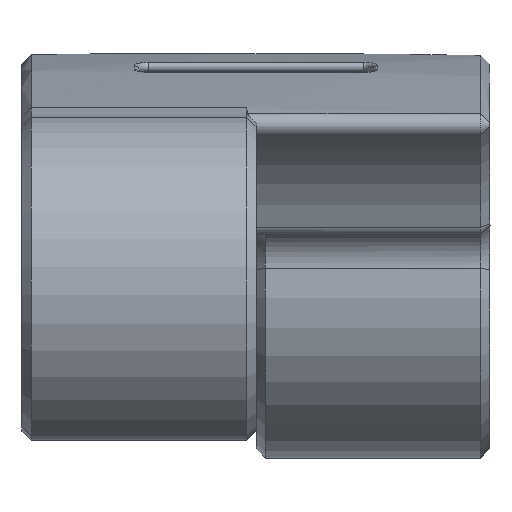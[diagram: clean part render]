
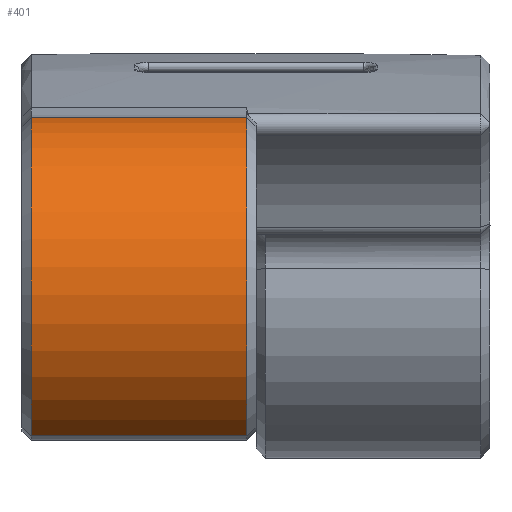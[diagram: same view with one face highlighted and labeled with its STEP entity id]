
A CAD part, front view. The second image highlights one B-rep face of the part: STEP entity #401.
In plain terms, the highlighted cylindrical face has radius 14.583 mm (diameter 29.165 mm), a partial arc.
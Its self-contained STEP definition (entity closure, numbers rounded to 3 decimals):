
#82 = DIRECTION ( 'NONE',  ( -1., 0., 0. ) ) ;
#241 = CYLINDRICAL_SURFACE ( 'NONE', #3236, 14.583 ) ;
#313 = CARTESIAN_POINT ( 'NONE',  ( -459.696, -70.336, 0.8 ) ) ;
#401 = ADVANCED_FACE ( 'NONE', ( #669 ), #241, .T. ) ;
#600 = DIRECTION ( 'NONE',  ( 0., 0., 1. ) ) ;
#618 = DIRECTION ( 'NONE',  ( 1., 0., 0. ) ) ;
#637 = VECTOR ( 'NONE', #3284, 1000. ) ;
#669 = FACE_OUTER_BOUND ( 'NONE', #1401, .T. ) ;
#715 = DIRECTION ( 'NONE',  ( 1., 0., 0. ) ) ;
#960 = ORIENTED_EDGE ( 'NONE', *, *, #1459, .F. ) ;
#1144 = DIRECTION ( 'NONE',  ( 0., 0., 1. ) ) ;
#1326 = CARTESIAN_POINT ( 'NONE',  ( -459.696, -77.575, -11.858 ) ) ;
#1401 = EDGE_LOOP ( 'NONE', ( #960, #3217, #1725, #2146 ) ) ;
#1449 = CARTESIAN_POINT ( 'NONE',  ( -445.481, -70.336, 0.8 ) ) ;
#1459 = EDGE_CURVE ( 'NONE', #3548, #3424, #3009, .T. ) ;
#1602 = VECTOR ( 'NONE', #715, 1000. ) ;
#1684 = EDGE_CURVE ( 'NONE', #3424, #3173, #1743, .T. ) ;
#1720 = DIRECTION ( 'NONE',  ( 1., 0., 0. ) ) ;
#1721 = CARTESIAN_POINT ( 'NONE',  ( -463.881, -70.336, 0.8 ) ) ;
#1725 = ORIENTED_EDGE ( 'NONE', *, *, #2529, .F. ) ;
#1743 = LINE ( 'NONE', #1326, #637 ) ;
#1800 = AXIS2_PLACEMENT_3D ( 'NONE', #1721, #82, #600 ) ;
#2042 = CIRCLE ( 'NONE', #1800, 14.583 ) ;
#2054 = AXIS2_PLACEMENT_3D ( 'NONE', #1449, #618, #2581 ) ;
#2146 = ORIENTED_EDGE ( 'NONE', *, *, #1684, .F. ) ;
#2283 = VERTEX_POINT ( 'NONE', #3160 ) ;
#2372 = CARTESIAN_POINT ( 'NONE',  ( -445.481, -69.39, 15.352 ) ) ;
#2411 = CARTESIAN_POINT ( 'NONE',  ( -454.681, -69.39, 15.352 ) ) ;
#2529 = EDGE_CURVE ( 'NONE', #3173, #2283, #2042, .T. ) ;
#2532 = LINE ( 'NONE', #2411, #1602 ) ;
#2581 = DIRECTION ( 'NONE',  ( 0., 0., 1. ) ) ;
#2991 = CARTESIAN_POINT ( 'NONE',  ( -445.481, -77.575, -11.858 ) ) ;
#3000 = CARTESIAN_POINT ( 'NONE',  ( -463.881, -77.575, -11.858 ) ) ;
#3009 = CIRCLE ( 'NONE', #2054, 14.583 ) ;
#3160 = CARTESIAN_POINT ( 'NONE',  ( -463.881, -69.39, 15.352 ) ) ;
#3173 = VERTEX_POINT ( 'NONE', #3000 ) ;
#3217 = ORIENTED_EDGE ( 'NONE', *, *, #3421, .F. ) ;
#3236 = AXIS2_PLACEMENT_3D ( 'NONE', #313, #1720, #1144 ) ;
#3284 = DIRECTION ( 'NONE',  ( -1., 0., 0. ) ) ;
#3421 = EDGE_CURVE ( 'NONE', #2283, #3548, #2532, .T. ) ;
#3424 = VERTEX_POINT ( 'NONE', #2991 ) ;
#3548 = VERTEX_POINT ( 'NONE', #2372 ) ;
